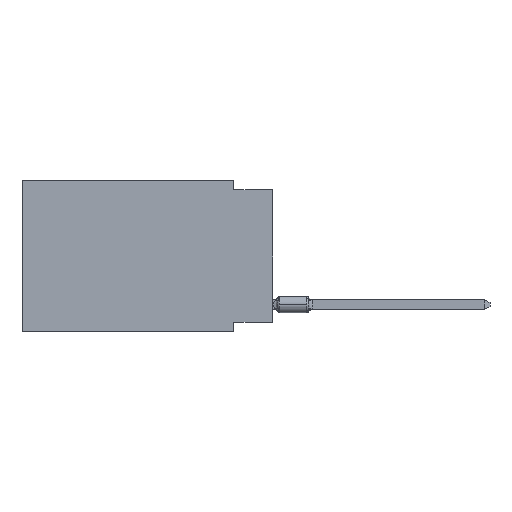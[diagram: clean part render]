
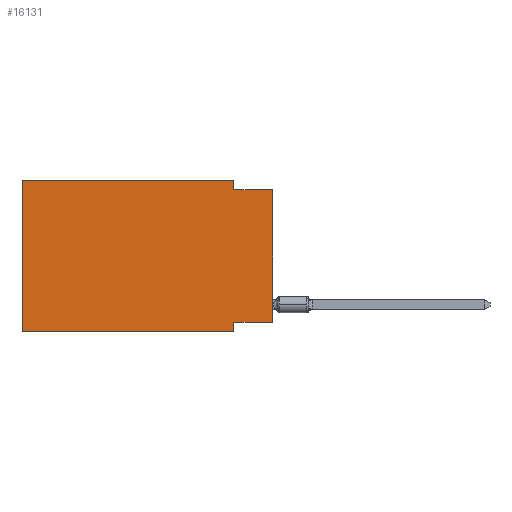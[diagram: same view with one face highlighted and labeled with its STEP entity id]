
A CAD part, left-side view. The second image highlights one B-rep face of the part: STEP entity #16131.
In plain terms, the highlighted planar face has unit normal (-1, 0, 0).
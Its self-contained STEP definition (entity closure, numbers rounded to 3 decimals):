
#324 = VECTOR ( 'NONE', #18186, 1000. ) ;
#663 = CARTESIAN_POINT ( 'NONE',  ( 0., 0., -0.635 ) ) ;
#723 = VERTEX_POINT ( 'NONE', #5271 ) ;
#893 = EDGE_CURVE ( 'NONE', #5352, #18374, #15322, .T. ) ;
#1092 = CARTESIAN_POINT ( 'NONE',  ( 0., 2.54, 0. ) ) ;
#1381 = VERTEX_POINT ( 'NONE', #15907 ) ;
#2115 = CARTESIAN_POINT ( 'NONE',  ( 0., 0., -9.271 ) ) ;
#2244 = ORIENTED_EDGE ( 'NONE', *, *, #7535, .T. ) ;
#2307 = VECTOR ( 'NONE', #10140, 1000. ) ;
#2342 = VECTOR ( 'NONE', #2750, 1000. ) ;
#2521 = ORIENTED_EDGE ( 'NONE', *, *, #893, .F. ) ;
#2750 = DIRECTION ( 'NONE',  ( 0., 0., 1. ) ) ;
#2808 = CARTESIAN_POINT ( 'NONE',  ( 0., 2.54, -9.906 ) ) ;
#2895 = CARTESIAN_POINT ( 'NONE',  ( 0., 0., -9.271 ) ) ;
#2897 = ORIENTED_EDGE ( 'NONE', *, *, #9522, .F. ) ;
#3043 = CARTESIAN_POINT ( 'NONE',  ( 0., 0., 0. ) ) ;
#3044 = LINE ( 'NONE', #18437, #11651 ) ;
#3407 = CARTESIAN_POINT ( 'NONE',  ( 0., 2.54, 0. ) ) ;
#4088 = EDGE_LOOP ( 'NONE', ( #2244, #2521, #12727, #2897, #18596, #14121, #17436, #6390 ) ) ;
#4109 = VECTOR ( 'NONE', #15131, 1000. ) ;
#5271 = CARTESIAN_POINT ( 'NONE',  ( 0., 16.383, -9.906 ) ) ;
#5274 = EDGE_CURVE ( 'NONE', #6836, #11217, #11059, .T. ) ;
#5352 = VERTEX_POINT ( 'NONE', #18608 ) ;
#5362 = DIRECTION ( 'NONE',  ( 0., 0., -1. ) ) ;
#5881 = LINE ( 'NONE', #10447, #324 ) ;
#6390 = ORIENTED_EDGE ( 'NONE', *, *, #5274, .F. ) ;
#6451 = VERTEX_POINT ( 'NONE', #10595 ) ;
#6836 = VERTEX_POINT ( 'NONE', #2895 ) ;
#6847 = FACE_OUTER_BOUND ( 'NONE', #4088, .T. ) ;
#6891 = CARTESIAN_POINT ( 'NONE',  ( 0., 2.54, -9.271 ) ) ;
#7070 = EDGE_CURVE ( 'NONE', #17461, #5352, #14597, .T. ) ;
#7535 = EDGE_CURVE ( 'NONE', #6836, #18374, #11995, .T. ) ;
#9522 = EDGE_CURVE ( 'NONE', #6451, #17461, #3044, .T. ) ;
#9935 = VECTOR ( 'NONE', #12256, 1000. ) ;
#10140 = DIRECTION ( 'NONE',  ( 0., 0., -1. ) ) ;
#10447 = CARTESIAN_POINT ( 'NONE',  ( 0., 16.383, -9.906 ) ) ;
#10595 = CARTESIAN_POINT ( 'NONE',  ( 0., 16.383, 0. ) ) ;
#11059 = LINE ( 'NONE', #2115, #14756 ) ;
#11157 = VECTOR ( 'NONE', #18837, 1000. ) ;
#11216 = DIRECTION ( 'NONE',  ( 1., 0., 0. ) ) ;
#11217 = VERTEX_POINT ( 'NONE', #6891 ) ;
#11651 = VECTOR ( 'NONE', #12193, 1000. ) ;
#11995 = LINE ( 'NONE', #3043, #2342 ) ;
#12193 = DIRECTION ( 'NONE',  ( 0., -1., 0. ) ) ;
#12256 = DIRECTION ( 'NONE',  ( 0., -1., 0. ) ) ;
#12727 = ORIENTED_EDGE ( 'NONE', *, *, #7070, .F. ) ;
#14121 = ORIENTED_EDGE ( 'NONE', *, *, #17665, .T. ) ;
#14258 = EDGE_CURVE ( 'NONE', #11217, #1381, #18003, .T. ) ;
#14491 = PLANE ( 'NONE',  #16278 ) ;
#14597 = LINE ( 'NONE', #1092, #2307 ) ;
#14756 = VECTOR ( 'NONE', #17194, 1000. ) ;
#15131 = DIRECTION ( 'NONE',  ( 0., 0., -1. ) ) ;
#15322 = LINE ( 'NONE', #15517, #9935 ) ;
#15517 = CARTESIAN_POINT ( 'NONE',  ( 0., 0., -0.635 ) ) ;
#15907 = CARTESIAN_POINT ( 'NONE',  ( 0., 2.54, -9.906 ) ) ;
#16131 = ADVANCED_FACE ( 'NONE', ( #6847 ), #14491, .F. ) ;
#16278 = AXIS2_PLACEMENT_3D ( 'NONE', #17664, #11216, #5362 ) ;
#17194 = DIRECTION ( 'NONE',  ( 0., 1., 0. ) ) ;
#17336 = CARTESIAN_POINT ( 'NONE',  ( 0., 16.383, 0. ) ) ;
#17436 = ORIENTED_EDGE ( 'NONE', *, *, #14258, .F. ) ;
#17461 = VERTEX_POINT ( 'NONE', #3407 ) ;
#17664 = CARTESIAN_POINT ( 'NONE',  ( 0., 16.383, 0. ) ) ;
#17665 = EDGE_CURVE ( 'NONE', #723, #1381, #5881, .T. ) ;
#18003 = LINE ( 'NONE', #2808, #4109 ) ;
#18186 = DIRECTION ( 'NONE',  ( 0., -1., 0. ) ) ;
#18374 = VERTEX_POINT ( 'NONE', #663 ) ;
#18377 = EDGE_CURVE ( 'NONE', #723, #6451, #19136, .T. ) ;
#18437 = CARTESIAN_POINT ( 'NONE',  ( 0., 16.383, 0. ) ) ;
#18596 = ORIENTED_EDGE ( 'NONE', *, *, #18377, .F. ) ;
#18608 = CARTESIAN_POINT ( 'NONE',  ( 0., 2.54, -0.635 ) ) ;
#18837 = DIRECTION ( 'NONE',  ( 0., 0., 1. ) ) ;
#19136 = LINE ( 'NONE', #17336, #11157 ) ;
